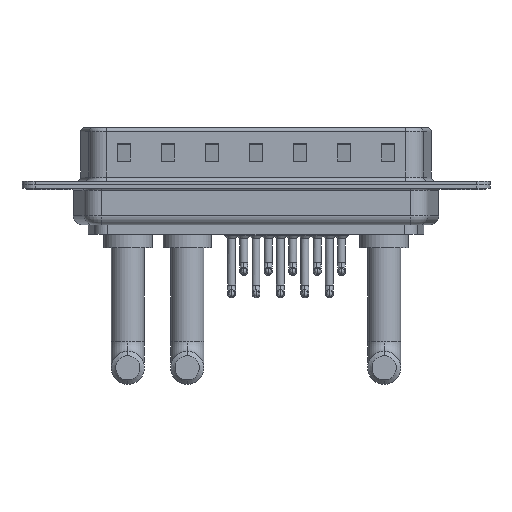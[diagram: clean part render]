
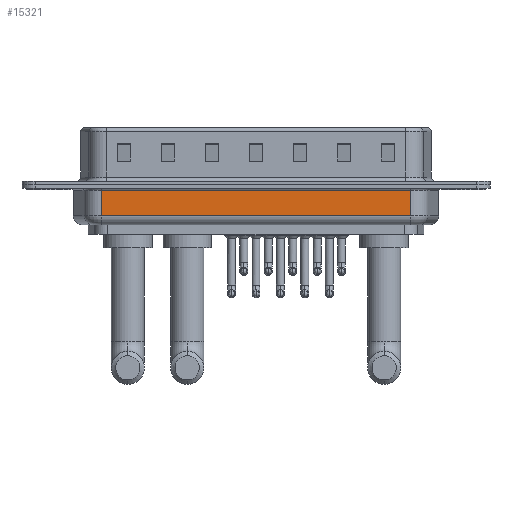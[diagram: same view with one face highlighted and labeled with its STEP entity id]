
A CAD part, front view. The second image highlights one B-rep face of the part: STEP entity #15321.
In plain terms, the highlighted planar face has unit normal (0, -1, 0).
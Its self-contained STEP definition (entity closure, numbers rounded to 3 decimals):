
#984 = ORIENTED_EDGE ( 'NONE', *, *, #986, .T. ) ;
#986 = EDGE_CURVE ( 'NONE', #3999, #6195, #4390, .T. ) ;
#1522 = VERTEX_POINT ( 'NONE', #15699 ) ;
#2483 = AXIS2_PLACEMENT_3D ( 'NONE', #9019, #6236, #4121 ) ;
#2737 = DIRECTION ( 'NONE',  ( 1., 0., 0. ) ) ;
#3437 = VECTOR ( 'NONE', #18740, 1000. ) ;
#3999 = VERTEX_POINT ( 'NONE', #9916 ) ;
#4121 = DIRECTION ( 'NONE',  ( 0., 0., 1. ) ) ;
#4390 = LINE ( 'NONE', #11164, #7931 ) ;
#5026 = EDGE_CURVE ( 'NONE', #3999, #20144, #5284, .T. ) ;
#5222 = LINE ( 'NONE', #13952, #10647 ) ;
#5284 = LINE ( 'NONE', #5616, #3437 ) ;
#5453 = CARTESIAN_POINT ( 'NONE',  ( 6.006, -5.35, -0.65 ) ) ;
#5616 = CARTESIAN_POINT ( 'NONE',  ( 6.006, -5.35, -4.5 ) ) ;
#5939 = EDGE_CURVE ( 'NONE', #6195, #1522, #7657, .T. ) ;
#6195 = VERTEX_POINT ( 'NONE', #21717 ) ;
#6236 = DIRECTION ( 'NONE',  ( 0., 1., 0. ) ) ;
#7566 = ORIENTED_EDGE ( 'NONE', *, *, #15682, .T. ) ;
#7657 = LINE ( 'NONE', #14682, #20069 ) ;
#7931 = VECTOR ( 'NONE', #2737, 1000. ) ;
#9019 = CARTESIAN_POINT ( 'NONE',  ( 6.006, -5.35, -4.5 ) ) ;
#9916 = CARTESIAN_POINT ( 'NONE',  ( 6.006, -5.35, -3.5 ) ) ;
#10209 = ORIENTED_EDGE ( 'NONE', *, *, #5939, .T. ) ;
#10647 = VECTOR ( 'NONE', #17460, 1000. ) ;
#11164 = CARTESIAN_POINT ( 'NONE',  ( 6.006, -5.35, -3.5 ) ) ;
#12344 = FACE_OUTER_BOUND ( 'NONE', #16337, .T. ) ;
#13952 = CARTESIAN_POINT ( 'NONE',  ( 6.006, -5.35, -0.65 ) ) ;
#14682 = CARTESIAN_POINT ( 'NONE',  ( 41.044, -5.35, -4.5 ) ) ;
#15321 = ADVANCED_FACE ( 'NONE', ( #12344 ), #19025, .F. ) ;
#15682 = EDGE_CURVE ( 'NONE', #1522, #20144, #5222, .T. ) ;
#15699 = CARTESIAN_POINT ( 'NONE',  ( 41.044, -5.35, -0.65 ) ) ;
#16337 = EDGE_LOOP ( 'NONE', ( #21149, #984, #10209, #7566 ) ) ;
#17460 = DIRECTION ( 'NONE',  ( -1., 0., 0. ) ) ;
#17981 = DIRECTION ( 'NONE',  ( 0., 0., 1. ) ) ;
#18740 = DIRECTION ( 'NONE',  ( 0., 0., 1. ) ) ;
#19025 = PLANE ( 'NONE',  #2483 ) ;
#20069 = VECTOR ( 'NONE', #17981, 1000. ) ;
#20144 = VERTEX_POINT ( 'NONE', #5453 ) ;
#21149 = ORIENTED_EDGE ( 'NONE', *, *, #5026, .F. ) ;
#21717 = CARTESIAN_POINT ( 'NONE',  ( 41.044, -5.35, -3.5 ) ) ;
